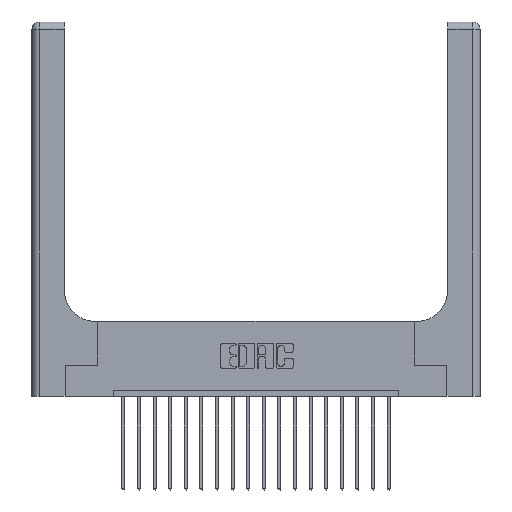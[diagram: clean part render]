
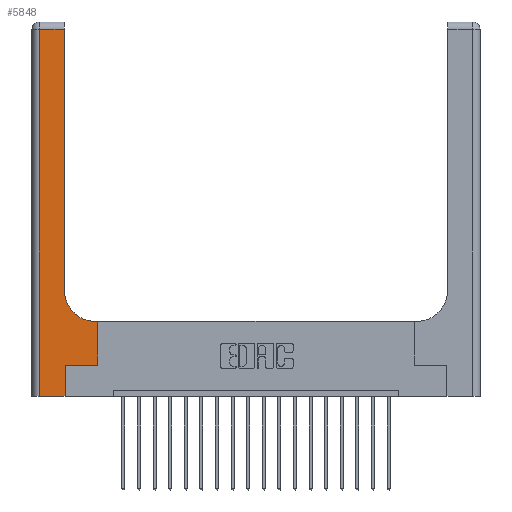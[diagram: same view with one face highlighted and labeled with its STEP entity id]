
A CAD part, top view. The second image highlights one B-rep face of the part: STEP entity #5848.
In plain terms, the highlighted planar face has unit normal (0, 0, 1).
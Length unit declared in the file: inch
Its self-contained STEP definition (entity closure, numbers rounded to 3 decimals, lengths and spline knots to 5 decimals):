
#94 = CARTESIAN_POINT ( 'NONE',  ( 0.26, 0.85, 0.37 ) ) ;
#261 = ORIENTED_EDGE ( 'NONE', *, *, #4266, .T. ) ;
#1051 = CARTESIAN_POINT ( 'NONE',  ( 0.06, 0., 0.37 ) ) ;
#1212 = DIRECTION ( 'NONE',  ( 1., 0., 0. ) ) ;
#1259 = EDGE_CURVE ( 'NONE', #3851, #1608, #9607, .T. ) ;
#1403 = LINE ( 'NONE', #18523, #7778 ) ;
#1405 = DIRECTION ( 'NONE',  ( -1., 0., 0. ) ) ;
#1543 = ORIENTED_EDGE ( 'NONE', *, *, #15632, .T. ) ;
#1608 = VERTEX_POINT ( 'NONE', #94 ) ;
#1747 = VECTOR ( 'NONE', #4657, 39.37008 ) ;
#1985 = CARTESIAN_POINT ( 'NONE',  ( 0.06, 2.94, 0.37 ) ) ;
#1997 = EDGE_CURVE ( 'NONE', #1608, #17740, #1403, .T. ) ;
#2225 = EDGE_CURVE ( 'NONE', #20007, #18508, #10102, .T. ) ;
#2408 = DIRECTION ( 'NONE',  ( -1., 0., 0. ) ) ;
#2598 = CARTESIAN_POINT ( 'NONE',  ( 0.265, 0., 0.37 ) ) ;
#2662 = CARTESIAN_POINT ( 'NONE',  ( 0.06, 3., 0.37 ) ) ;
#2765 = EDGE_LOOP ( 'NONE', ( #4359, #18855, #261, #6434, #4395, #1543, #10775, #4286, #8841 ) ) ;
#2891 = CARTESIAN_POINT ( 'NONE',  ( 0.51, 0.6, 0.37 ) ) ;
#3095 = PLANE ( 'NONE',  #13660 ) ;
#3194 = FACE_OUTER_BOUND ( 'NONE', #2765, .T. ) ;
#3793 = AXIS2_PLACEMENT_3D ( 'NONE', #17178, #4930, #14622 ) ;
#3851 = VERTEX_POINT ( 'NONE', #2891 ) ;
#4041 = CARTESIAN_POINT ( 'NONE',  ( 0.528, 0.25, 0.37 ) ) ;
#4266 = EDGE_CURVE ( 'NONE', #9361, #20007, #19976, .T. ) ;
#4286 = ORIENTED_EDGE ( 'NONE', *, *, #12832, .T. ) ;
#4359 = ORIENTED_EDGE ( 'NONE', *, *, #1997, .T. ) ;
#4395 = ORIENTED_EDGE ( 'NONE', *, *, #9974, .T. ) ;
#4657 = DIRECTION ( 'NONE',  ( 0., 1., 0. ) ) ;
#4930 = DIRECTION ( 'NONE',  ( 0., 0., -1. ) ) ;
#5654 = CARTESIAN_POINT ( 'NONE',  ( 0., 0., 0.37 ) ) ;
#5848 = ADVANCED_FACE ( 'NONE', ( #3194 ), #3095, .F. ) ;
#5987 = VERTEX_POINT ( 'NONE', #14537 ) ;
#6434 = ORIENTED_EDGE ( 'NONE', *, *, #2225, .T. ) ;
#6581 = CARTESIAN_POINT ( 'NONE',  ( 0., 2.94, 0.37 ) ) ;
#6976 = LINE ( 'NONE', #4041, #12241 ) ;
#7201 = CARTESIAN_POINT ( 'NONE',  ( 0.265, 0.25, 0.37 ) ) ;
#7275 = DIRECTION ( 'NONE',  ( 0., 1., 0. ) ) ;
#7778 = VECTOR ( 'NONE', #13763, 39.37008 ) ;
#8006 = VECTOR ( 'NONE', #1212, 39.37008 ) ;
#8396 = VECTOR ( 'NONE', #16292, 39.37008 ) ;
#8841 = ORIENTED_EDGE ( 'NONE', *, *, #1259, .T. ) ;
#9243 = CARTESIAN_POINT ( 'NONE',  ( 0.528, 0.25, 0.37 ) ) ;
#9361 = VERTEX_POINT ( 'NONE', #1985 ) ;
#9607 = CIRCLE ( 'NONE', #3793, 0.25 ) ;
#9608 = LINE ( 'NONE', #18524, #1747 ) ;
#9974 = EDGE_CURVE ( 'NONE', #18508, #5987, #9608, .T. ) ;
#10055 = VECTOR ( 'NONE', #11971, 39.37008 ) ;
#10064 = EDGE_CURVE ( 'NONE', #17740, #9361, #13148, .T. ) ;
#10102 = LINE ( 'NONE', #5654, #8396 ) ;
#10235 = VECTOR ( 'NONE', #1405, 39.37008 ) ;
#10425 = CARTESIAN_POINT ( 'NONE',  ( 0.26, 0.6, 0.37 ) ) ;
#10775 = ORIENTED_EDGE ( 'NONE', *, *, #16833, .T. ) ;
#11456 = VECTOR ( 'NONE', #2408, 39.37008 ) ;
#11971 = DIRECTION ( 'NONE',  ( 0., -1., 0. ) ) ;
#12241 = VECTOR ( 'NONE', #7275, 39.37008 ) ;
#12402 = CARTESIAN_POINT ( 'NONE',  ( 0., 3., 0.37 ) ) ;
#12477 = VERTEX_POINT ( 'NONE', #16907 ) ;
#12832 = EDGE_CURVE ( 'NONE', #12477, #3851, #15892, .T. ) ;
#13148 = LINE ( 'NONE', #6581, #11456 ) ;
#13660 = AXIS2_PLACEMENT_3D ( 'NONE', #12402, #17072, #15455 ) ;
#13763 = DIRECTION ( 'NONE',  ( 0., 1., 0. ) ) ;
#14537 = CARTESIAN_POINT ( 'NONE',  ( 0.265, 0.25, 0.37 ) ) ;
#14622 = DIRECTION ( 'NONE',  ( 1., 0., 0. ) ) ;
#14901 = LINE ( 'NONE', #7201, #8006 ) ;
#15455 = DIRECTION ( 'NONE',  ( -1., 0., 0. ) ) ;
#15632 = EDGE_CURVE ( 'NONE', #5987, #20029, #14901, .T. ) ;
#15892 = LINE ( 'NONE', #10425, #10235 ) ;
#16292 = DIRECTION ( 'NONE',  ( 1., 0., 0. ) ) ;
#16833 = EDGE_CURVE ( 'NONE', #20029, #12477, #6976, .T. ) ;
#16907 = CARTESIAN_POINT ( 'NONE',  ( 0.528, 0.6, 0.37 ) ) ;
#17072 = DIRECTION ( 'NONE',  ( 0., 0., -1. ) ) ;
#17178 = CARTESIAN_POINT ( 'NONE',  ( 0.51, 0.85, 0.37 ) ) ;
#17740 = VERTEX_POINT ( 'NONE', #18258 ) ;
#18258 = CARTESIAN_POINT ( 'NONE',  ( 0.26, 2.94, 0.37 ) ) ;
#18508 = VERTEX_POINT ( 'NONE', #2598 ) ;
#18523 = CARTESIAN_POINT ( 'NONE',  ( 0.26, 3., 0.37 ) ) ;
#18524 = CARTESIAN_POINT ( 'NONE',  ( 0.265, 0., 0.37 ) ) ;
#18855 = ORIENTED_EDGE ( 'NONE', *, *, #10064, .T. ) ;
#19976 = LINE ( 'NONE', #2662, #10055 ) ;
#20007 = VERTEX_POINT ( 'NONE', #1051 ) ;
#20029 = VERTEX_POINT ( 'NONE', #9243 ) ;
